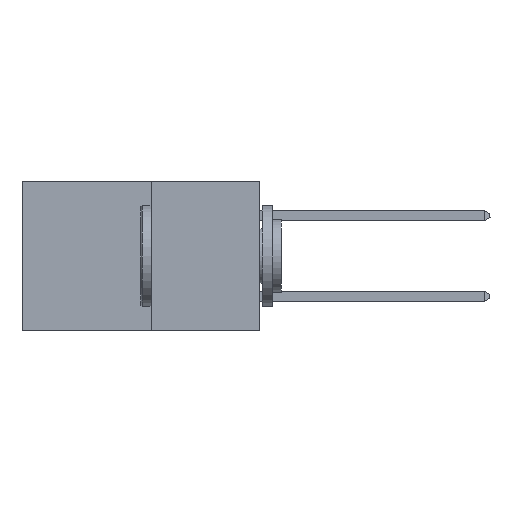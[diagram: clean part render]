
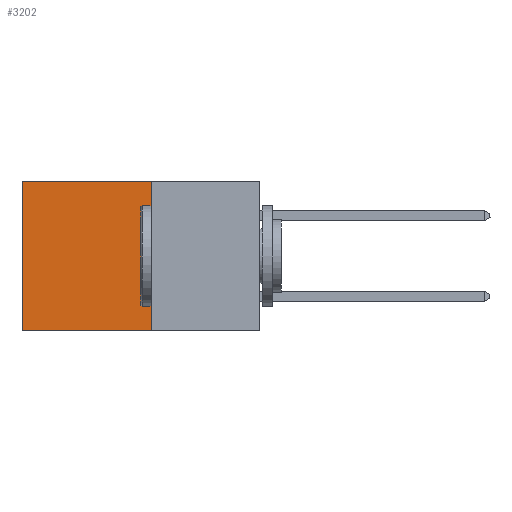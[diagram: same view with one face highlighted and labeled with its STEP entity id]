
A CAD part, left-side view. The second image highlights one B-rep face of the part: STEP entity #3202.
In plain terms, the highlighted planar face has unit normal (-1, 0, 0).
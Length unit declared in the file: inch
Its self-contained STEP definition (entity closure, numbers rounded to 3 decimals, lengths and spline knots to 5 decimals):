
#493 = CARTESIAN_POINT ( 'NONE',  ( 0.277, 0.59, -0.37 ) ) ;
#1062 = EDGE_CURVE ( 'NONE', #17160, #2418, #19062, .T. ) ;
#1877 = CARTESIAN_POINT ( 'NONE',  ( 0.277, 0.27, -0.37 ) ) ;
#1910 = CARTESIAN_POINT ( 'NONE',  ( 0.277, 0.27, -0.37 ) ) ;
#2418 = VERTEX_POINT ( 'NONE', #11963 ) ;
#2533 = EDGE_CURVE ( 'NONE', #16440, #4878, #11953, .T. ) ;
#3033 = CARTESIAN_POINT ( 'NONE',  ( 0.277, 0.59, -0.37 ) ) ;
#3202 = ADVANCED_FACE ( 'NONE', ( #11661 ), #10766, .F. ) ;
#3296 = DIRECTION ( 'NONE',  ( 0., 0., -1. ) ) ;
#4485 = ORIENTED_EDGE ( 'NONE', *, *, #19575, .T. ) ;
#4610 = CARTESIAN_POINT ( 'NONE',  ( 0.277, 0.27, 0. ) ) ;
#4707 = DIRECTION ( 'NONE',  ( 0., 0., -1. ) ) ;
#4878 = VERTEX_POINT ( 'NONE', #3033 ) ;
#5221 = VECTOR ( 'NONE', #18330, 39.37008 ) ;
#6930 = VECTOR ( 'NONE', #11727, 39.37008 ) ;
#7929 = DIRECTION ( 'NONE',  ( 0., 0., -1. ) ) ;
#7965 = DIRECTION ( 'NONE',  ( 1., 0., 0. ) ) ;
#10766 = PLANE ( 'NONE',  #11936 ) ;
#11199 = ORIENTED_EDGE ( 'NONE', *, *, #2533, .T. ) ;
#11444 = VECTOR ( 'NONE', #4707, 39.37008 ) ;
#11661 = FACE_OUTER_BOUND ( 'NONE', #15286, .T. ) ;
#11679 = ORIENTED_EDGE ( 'NONE', *, *, #1062, .F. ) ;
#11727 = DIRECTION ( 'NONE',  ( 0., 1., 0. ) ) ;
#11787 = CARTESIAN_POINT ( 'NONE',  ( 0.277, 0.27, -0.37 ) ) ;
#11936 = AXIS2_PLACEMENT_3D ( 'NONE', #1910, #7965, #7929 ) ;
#11953 = LINE ( 'NONE', #493, #11444 ) ;
#11963 = CARTESIAN_POINT ( 'NONE',  ( 0.277, 0.27, -0.37 ) ) ;
#13351 = LINE ( 'NONE', #4610, #5221 ) ;
#14622 = LINE ( 'NONE', #11787, #6930 ) ;
#15268 = ORIENTED_EDGE ( 'NONE', *, *, #17640, .F. ) ;
#15277 = CARTESIAN_POINT ( 'NONE',  ( 0.277, 0.27, 0. ) ) ;
#15286 = EDGE_LOOP ( 'NONE', ( #11199, #15268, #11679, #4485 ) ) ;
#16029 = VECTOR ( 'NONE', #3296, 39.37008 ) ;
#16440 = VERTEX_POINT ( 'NONE', #18071 ) ;
#17160 = VERTEX_POINT ( 'NONE', #15277 ) ;
#17640 = EDGE_CURVE ( 'NONE', #2418, #4878, #14622, .T. ) ;
#18071 = CARTESIAN_POINT ( 'NONE',  ( 0.277, 0.59, 0. ) ) ;
#18330 = DIRECTION ( 'NONE',  ( 0., 1., 0. ) ) ;
#19062 = LINE ( 'NONE', #1877, #16029 ) ;
#19575 = EDGE_CURVE ( 'NONE', #17160, #16440, #13351, .T. ) ;
